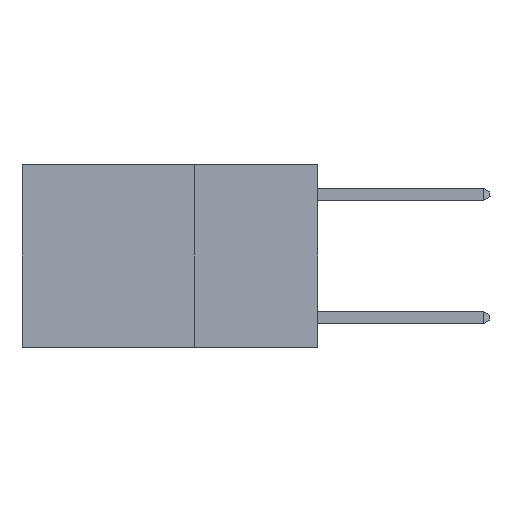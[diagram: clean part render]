
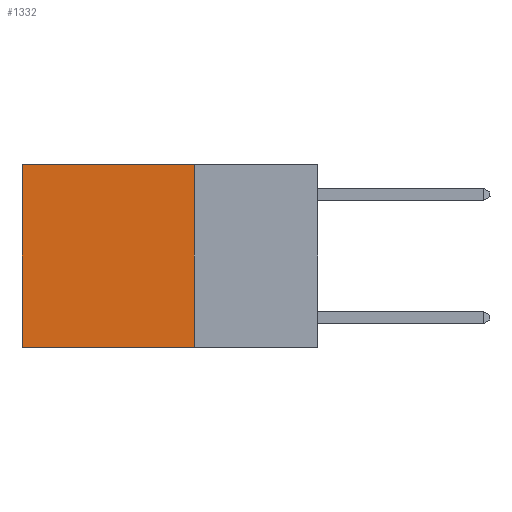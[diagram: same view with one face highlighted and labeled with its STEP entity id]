
A CAD part, left-side view. The second image highlights one B-rep face of the part: STEP entity #1332.
In plain terms, the highlighted planar face has unit normal (-1, 0, 0).
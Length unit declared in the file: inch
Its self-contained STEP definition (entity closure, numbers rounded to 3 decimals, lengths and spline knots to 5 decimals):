
#74 = ORIENTED_EDGE ( 'NONE', *, *, #7584, .T. ) ;
#460 = VERTEX_POINT ( 'NONE', #10249 ) ;
#464 = ORIENTED_EDGE ( 'NONE', *, *, #10242, .F. ) ;
#1332 = ADVANCED_FACE ( 'NONE', ( #2901 ), #4340, .F. ) ;
#1680 = LINE ( 'NONE', #7996, #4356 ) ;
#1792 = DIRECTION ( 'NONE',  ( 0., 0., -1. ) ) ;
#2587 = EDGE_CURVE ( 'NONE', #3752, #460, #1680, .T. ) ;
#2662 = EDGE_CURVE ( 'NONE', #3752, #4030, #4350, .T. ) ;
#2778 = LINE ( 'NONE', #5917, #2780 ) ;
#2780 = VECTOR ( 'NONE', #5956, 39.37008 ) ;
#2901 = FACE_OUTER_BOUND ( 'NONE', #9731, .T. ) ;
#3582 = CARTESIAN_POINT ( 'NONE',  ( 0.2625, 0.25, 0. ) ) ;
#3752 = VERTEX_POINT ( 'NONE', #4371 ) ;
#3971 = VERTEX_POINT ( 'NONE', #8689 ) ;
#4030 = VERTEX_POINT ( 'NONE', #5091 ) ;
#4340 = PLANE ( 'NONE',  #7484 ) ;
#4350 = LINE ( 'NONE', #5806, #9500 ) ;
#4356 = VECTOR ( 'NONE', #1792, 39.37008 ) ;
#4371 = CARTESIAN_POINT ( 'NONE',  ( 0.2625, 0.25, 0. ) ) ;
#5091 = CARTESIAN_POINT ( 'NONE',  ( 0.2625, 0.6, 0. ) ) ;
#5164 = DIRECTION ( 'NONE',  ( 1., 0., 0. ) ) ;
#5244 = ORIENTED_EDGE ( 'NONE', *, *, #2587, .F. ) ;
#5740 = LINE ( 'NONE', #5786, #10182 ) ;
#5786 = CARTESIAN_POINT ( 'NONE',  ( 0.2625, 0.25, -0.37 ) ) ;
#5806 = CARTESIAN_POINT ( 'NONE',  ( 0.2625, 0.25, 0. ) ) ;
#5917 = CARTESIAN_POINT ( 'NONE',  ( 0.2625, 0.6, 0. ) ) ;
#5956 = DIRECTION ( 'NONE',  ( 0., 0., -1. ) ) ;
#6637 = DIRECTION ( 'NONE',  ( 0., 1., 0. ) ) ;
#7019 = ORIENTED_EDGE ( 'NONE', *, *, #2662, .T. ) ;
#7484 = AXIS2_PLACEMENT_3D ( 'NONE', #3582, #5164, #8446 ) ;
#7584 = EDGE_CURVE ( 'NONE', #4030, #3971, #2778, .T. ) ;
#7996 = CARTESIAN_POINT ( 'NONE',  ( 0.2625, 0.25, 0. ) ) ;
#8446 = DIRECTION ( 'NONE',  ( 0., 0., -1. ) ) ;
#8689 = CARTESIAN_POINT ( 'NONE',  ( 0.2625, 0.6, -0.37 ) ) ;
#8928 = DIRECTION ( 'NONE',  ( 0., 1., 0. ) ) ;
#9500 = VECTOR ( 'NONE', #6637, 39.37008 ) ;
#9731 = EDGE_LOOP ( 'NONE', ( #74, #464, #5244, #7019 ) ) ;
#10182 = VECTOR ( 'NONE', #8928, 39.37008 ) ;
#10242 = EDGE_CURVE ( 'NONE', #460, #3971, #5740, .T. ) ;
#10249 = CARTESIAN_POINT ( 'NONE',  ( 0.2625, 0.25, -0.37 ) ) ;
